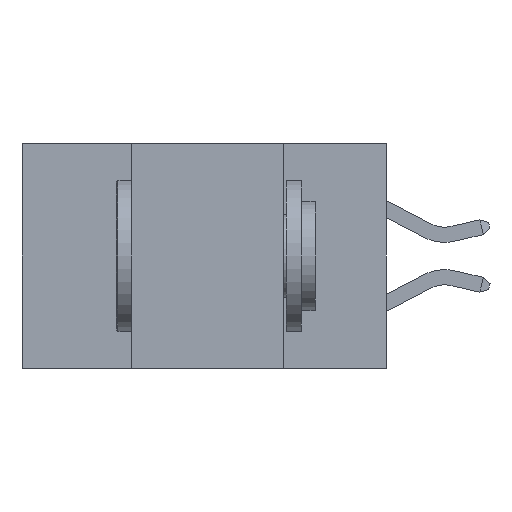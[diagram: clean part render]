
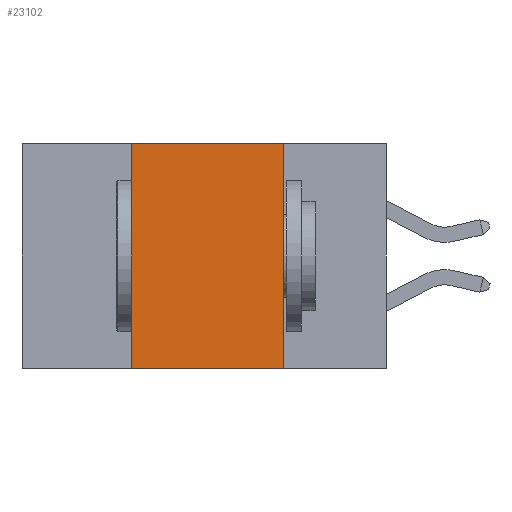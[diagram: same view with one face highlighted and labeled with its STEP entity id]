
A CAD part, left-side view. The second image highlights one B-rep face of the part: STEP entity #23102.
In plain terms, the highlighted planar face has unit normal (-1, 0, 0).
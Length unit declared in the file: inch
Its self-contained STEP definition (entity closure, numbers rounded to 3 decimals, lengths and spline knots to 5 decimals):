
#35 = VERTEX_POINT ( 'NONE', #12288 ) ;
#335 = VERTEX_POINT ( 'NONE', #5958 ) ;
#393 = LINE ( 'NONE', #11057, #4584 ) ;
#1093 = FACE_OUTER_BOUND ( 'NONE', #20447, .T. ) ;
#2054 = EDGE_CURVE ( 'NONE', #19651, #335, #23853, .T. ) ;
#2363 = ORIENTED_EDGE ( 'NONE', *, *, #21560, .F. ) ;
#2495 = VECTOR ( 'NONE', #21722, 39.37008 ) ;
#2892 = DIRECTION ( 'NONE',  ( 0., 0., 1. ) ) ;
#3011 = ORIENTED_EDGE ( 'NONE', *, *, #25389, .T. ) ;
#3349 = CARTESIAN_POINT ( 'NONE',  ( 0., 0.17, -0.37 ) ) ;
#4293 = CARTESIAN_POINT ( 'NONE',  ( 0., 0.6, 0. ) ) ;
#4584 = VECTOR ( 'NONE', #2892, 39.37008 ) ;
#4820 = EDGE_CURVE ( 'NONE', #7641, #19651, #23843, .T. ) ;
#5373 = CARTESIAN_POINT ( 'NONE',  ( 0., 0.42, 0. ) ) ;
#5958 = CARTESIAN_POINT ( 'NONE',  ( 0., 0.17, -0.37 ) ) ;
#6535 = ORIENTED_EDGE ( 'NONE', *, *, #2054, .F. ) ;
#7641 = VERTEX_POINT ( 'NONE', #5373 ) ;
#7803 = DIRECTION ( 'NONE',  ( 0., -1., 0. ) ) ;
#7935 = VECTOR ( 'NONE', #7803, 39.37008 ) ;
#7992 = CARTESIAN_POINT ( 'NONE',  ( 0., 0.6, 0. ) ) ;
#10476 = DIRECTION ( 'NONE',  ( 1., 0., 0. ) ) ;
#10732 = AXIS2_PLACEMENT_3D ( 'NONE', #4293, #10476, #24337 ) ;
#11030 = DIRECTION ( 'NONE',  ( 0., -1., 0. ) ) ;
#11057 = CARTESIAN_POINT ( 'NONE',  ( 0., 0.42, -0.37 ) ) ;
#12288 = CARTESIAN_POINT ( 'NONE',  ( 0., 0.42, -0.37 ) ) ;
#13165 = LINE ( 'NONE', #24859, #18481 ) ;
#16542 = PLANE ( 'NONE',  #10732 ) ;
#17145 = CARTESIAN_POINT ( 'NONE',  ( 0., 0.17, 0. ) ) ;
#17973 = ORIENTED_EDGE ( 'NONE', *, *, #4820, .F. ) ;
#18481 = VECTOR ( 'NONE', #11030, 39.37008 ) ;
#19651 = VERTEX_POINT ( 'NONE', #17145 ) ;
#20447 = EDGE_LOOP ( 'NONE', ( #6535, #17973, #2363, #3011 ) ) ;
#21560 = EDGE_CURVE ( 'NONE', #35, #7641, #393, .T. ) ;
#21722 = DIRECTION ( 'NONE',  ( 0., 0., -1. ) ) ;
#23102 = ADVANCED_FACE ( 'NONE', ( #1093 ), #16542, .F. ) ;
#23843 = LINE ( 'NONE', #7992, #7935 ) ;
#23853 = LINE ( 'NONE', #3349, #2495 ) ;
#24337 = DIRECTION ( 'NONE',  ( 0., 0., -1. ) ) ;
#24859 = CARTESIAN_POINT ( 'NONE',  ( 0., 0.6, -0.37 ) ) ;
#25389 = EDGE_CURVE ( 'NONE', #35, #335, #13165, .T. ) ;
